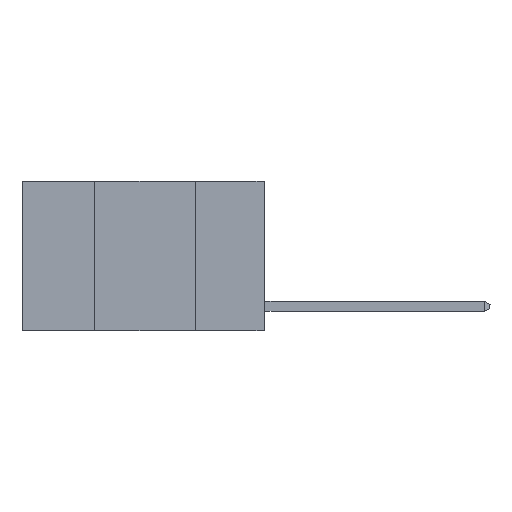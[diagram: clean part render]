
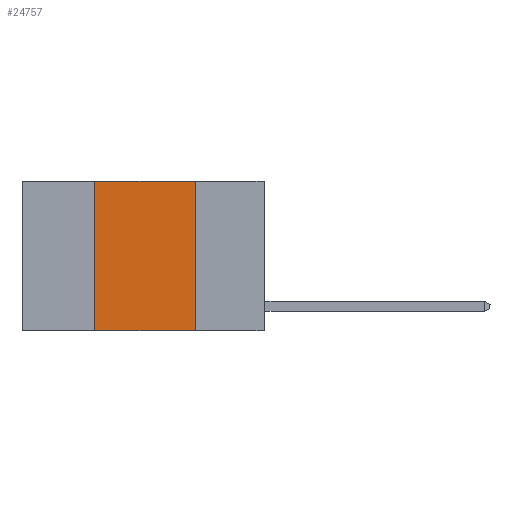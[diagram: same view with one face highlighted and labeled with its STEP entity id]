
A CAD part, left-side view. The second image highlights one B-rep face of the part: STEP entity #24757.
In plain terms, the highlighted planar face has unit normal (-1, 0, 0).
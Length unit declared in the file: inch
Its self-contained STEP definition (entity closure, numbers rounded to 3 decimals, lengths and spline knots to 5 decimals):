
#483 = EDGE_LOOP ( 'NONE', ( #18905, #23742, #12116, #14061 ) ) ;
#832 = VECTOR ( 'NONE', #22868, 39.37008 ) ;
#1087 = CARTESIAN_POINT ( 'NONE',  ( 0., 0.42, 0. ) ) ;
#2602 = LINE ( 'NONE', #19786, #23950 ) ;
#3996 = LINE ( 'NONE', #10909, #832 ) ;
#4018 = VECTOR ( 'NONE', #17541, 39.37008 ) ;
#4042 = CARTESIAN_POINT ( 'NONE',  ( 0., 0.6, 0. ) ) ;
#4135 = DIRECTION ( 'NONE',  ( 1., 0., 0. ) ) ;
#4905 = VECTOR ( 'NONE', #11460, 39.37008 ) ;
#6021 = DIRECTION ( 'NONE',  ( 0., -1., 0. ) ) ;
#6575 = LINE ( 'NONE', #25514, #4018 ) ;
#8551 = VERTEX_POINT ( 'NONE', #23317 ) ;
#9812 = EDGE_CURVE ( 'NONE', #20318, #18839, #3996, .T. ) ;
#10909 = CARTESIAN_POINT ( 'NONE',  ( 0., 0.42, 0. ) ) ;
#11460 = DIRECTION ( 'NONE',  ( 0., 0., -1. ) ) ;
#12116 = ORIENTED_EDGE ( 'NONE', *, *, #9812, .F. ) ;
#13383 = VERTEX_POINT ( 'NONE', #22105 ) ;
#14061 = ORIENTED_EDGE ( 'NONE', *, *, #14959, .T. ) ;
#14523 = CARTESIAN_POINT ( 'NONE',  ( 0., 0.42, -0.37 ) ) ;
#14959 = EDGE_CURVE ( 'NONE', #20318, #8551, #2602, .T. ) ;
#17050 = LINE ( 'NONE', #23608, #4905 ) ;
#17541 = DIRECTION ( 'NONE',  ( 0., -1., 0. ) ) ;
#18383 = EDGE_CURVE ( 'NONE', #18839, #13383, #6575, .T. ) ;
#18506 = AXIS2_PLACEMENT_3D ( 'NONE', #4042, #4135, #24768 ) ;
#18839 = VERTEX_POINT ( 'NONE', #1087 ) ;
#18905 = ORIENTED_EDGE ( 'NONE', *, *, #19385, .F. ) ;
#18929 = FACE_OUTER_BOUND ( 'NONE', #483, .T. ) ;
#19385 = EDGE_CURVE ( 'NONE', #13383, #8551, #17050, .T. ) ;
#19786 = CARTESIAN_POINT ( 'NONE',  ( 0., 0.6, -0.37 ) ) ;
#20318 = VERTEX_POINT ( 'NONE', #14523 ) ;
#22105 = CARTESIAN_POINT ( 'NONE',  ( 0., 0.17, 0. ) ) ;
#22668 = PLANE ( 'NONE',  #18506 ) ;
#22868 = DIRECTION ( 'NONE',  ( 0., 0., 1. ) ) ;
#23317 = CARTESIAN_POINT ( 'NONE',  ( 0., 0.17, -0.37 ) ) ;
#23608 = CARTESIAN_POINT ( 'NONE',  ( 0., 0.17, 0. ) ) ;
#23742 = ORIENTED_EDGE ( 'NONE', *, *, #18383, .F. ) ;
#23950 = VECTOR ( 'NONE', #6021, 39.37008 ) ;
#24757 = ADVANCED_FACE ( 'NONE', ( #18929 ), #22668, .F. ) ;
#24768 = DIRECTION ( 'NONE',  ( 0., 0., -1. ) ) ;
#25514 = CARTESIAN_POINT ( 'NONE',  ( 0., 0.6, 0. ) ) ;
